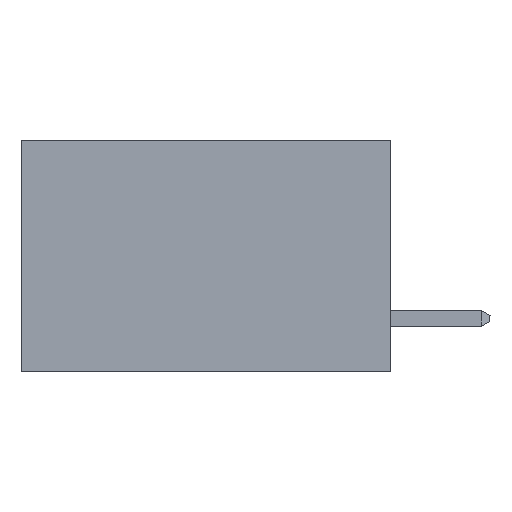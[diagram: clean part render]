
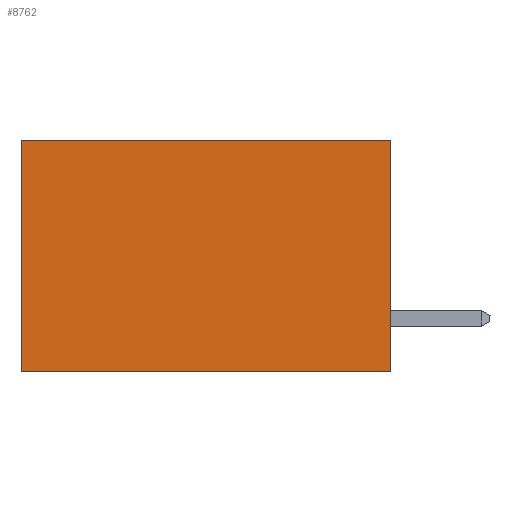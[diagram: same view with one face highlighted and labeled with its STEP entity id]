
A CAD part, left-side view. The second image highlights one B-rep face of the part: STEP entity #8762.
In plain terms, the highlighted planar face has unit normal (-1, 0, 0).
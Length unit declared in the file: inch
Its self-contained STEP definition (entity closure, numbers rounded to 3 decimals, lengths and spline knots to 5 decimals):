
#187 = LINE ( 'NONE', #1938, #2292 ) ;
#355 = VERTEX_POINT ( 'NONE', #5535 ) ;
#488 = VERTEX_POINT ( 'NONE', #7010 ) ;
#699 = LINE ( 'NONE', #5846, #4277 ) ;
#795 = FACE_OUTER_BOUND ( 'NONE', #5385, .T. ) ;
#892 = AXIS2_PLACEMENT_3D ( 'NONE', #3621, #8229, #4364 ) ;
#1366 = VERTEX_POINT ( 'NONE', #3498 ) ;
#1590 = VERTEX_POINT ( 'NONE', #8532 ) ;
#1640 = DIRECTION ( 'NONE',  ( 0., 1., 0. ) ) ;
#1938 = CARTESIAN_POINT ( 'NONE',  ( 0.277, 0., 0. ) ) ;
#2079 = ORIENTED_EDGE ( 'NONE', *, *, #6755, .F. ) ;
#2292 = VECTOR ( 'NONE', #1640, 39.37008 ) ;
#3498 = CARTESIAN_POINT ( 'NONE',  ( 0.277, 0.59, 0. ) ) ;
#3621 = CARTESIAN_POINT ( 'NONE',  ( 0.277, 0., -0.37 ) ) ;
#3799 = ORIENTED_EDGE ( 'NONE', *, *, #4383, .T. ) ;
#4057 = ORIENTED_EDGE ( 'NONE', *, *, #4675, .T. ) ;
#4277 = VECTOR ( 'NONE', #8806, 39.37008 ) ;
#4364 = DIRECTION ( 'NONE',  ( 0., 0., -1. ) ) ;
#4383 = EDGE_CURVE ( 'NONE', #1366, #1590, #6145, .T. ) ;
#4445 = DIRECTION ( 'NONE',  ( 0., 0., -1. ) ) ;
#4675 = EDGE_CURVE ( 'NONE', #355, #1366, #187, .T. ) ;
#4740 = CARTESIAN_POINT ( 'NONE',  ( 0.277, 0.59, -0.37 ) ) ;
#5103 = CARTESIAN_POINT ( 'NONE',  ( 0.277, 0., -0.37 ) ) ;
#5385 = EDGE_LOOP ( 'NONE', ( #3799, #5753, #2079, #4057 ) ) ;
#5535 = CARTESIAN_POINT ( 'NONE',  ( 0.277, 0., 0. ) ) ;
#5753 = ORIENTED_EDGE ( 'NONE', *, *, #6798, .F. ) ;
#5763 = DIRECTION ( 'NONE',  ( 0., 0., -1. ) ) ;
#5846 = CARTESIAN_POINT ( 'NONE',  ( 0.277, 0., -0.37 ) ) ;
#6145 = LINE ( 'NONE', #4740, #7598 ) ;
#6561 = VECTOR ( 'NONE', #5763, 39.37008 ) ;
#6755 = EDGE_CURVE ( 'NONE', #355, #488, #8141, .T. ) ;
#6798 = EDGE_CURVE ( 'NONE', #488, #1590, #699, .T. ) ;
#7010 = CARTESIAN_POINT ( 'NONE',  ( 0.277, 0., -0.37 ) ) ;
#7598 = VECTOR ( 'NONE', #4445, 39.37008 ) ;
#7665 = PLANE ( 'NONE',  #892 ) ;
#8141 = LINE ( 'NONE', #5103, #6561 ) ;
#8229 = DIRECTION ( 'NONE',  ( 1., 0., 0. ) ) ;
#8532 = CARTESIAN_POINT ( 'NONE',  ( 0.277, 0.59, -0.37 ) ) ;
#8762 = ADVANCED_FACE ( 'NONE', ( #795 ), #7665, .F. ) ;
#8806 = DIRECTION ( 'NONE',  ( 0., 1., 0. ) ) ;
